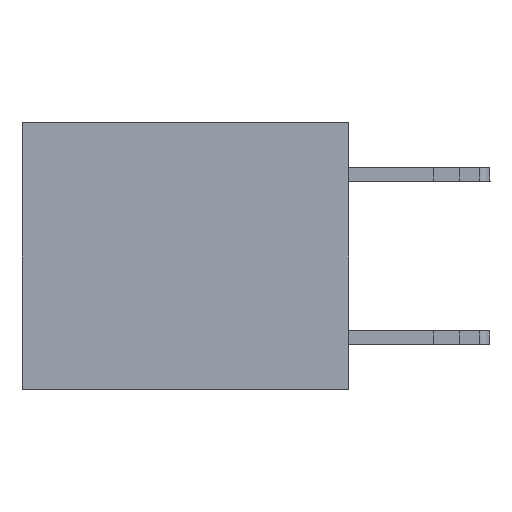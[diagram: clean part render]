
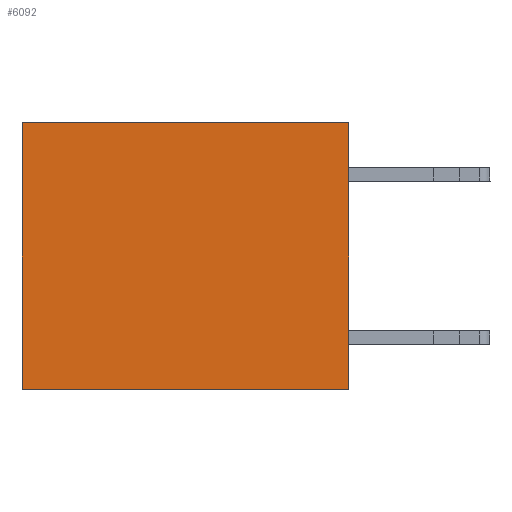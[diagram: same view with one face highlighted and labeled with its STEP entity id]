
A CAD part, left-side view. The second image highlights one B-rep face of the part: STEP entity #6092.
In plain terms, the highlighted planar face has unit normal (-1, 0, 0).
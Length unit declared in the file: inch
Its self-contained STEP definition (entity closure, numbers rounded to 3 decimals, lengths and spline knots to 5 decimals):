
#1588 = VERTEX_POINT ( 'NONE', #6888 ) ;
#2397 = EDGE_CURVE ( 'NONE', #4561, #4351, #5416, .T. ) ;
#2627 = CARTESIAN_POINT ( 'NONE',  ( 0.3165, 0., -0.49 ) ) ;
#3205 = VECTOR ( 'NONE', #15826, 39.37008 ) ;
#3655 = DIRECTION ( 'NONE',  ( 0., 0., -1. ) ) ;
#4344 = ORIENTED_EDGE ( 'NONE', *, *, #4669, .F. ) ;
#4351 = VERTEX_POINT ( 'NONE', #10273 ) ;
#4561 = VERTEX_POINT ( 'NONE', #13708 ) ;
#4669 = EDGE_CURVE ( 'NONE', #1588, #4351, #12256, .T. ) ;
#5416 = LINE ( 'NONE', #12578, #13364 ) ;
#5904 = EDGE_CURVE ( 'NONE', #9114, #1588, #15426, .T. ) ;
#6092 = ADVANCED_FACE ( 'NONE', ( #16741 ), #17981, .F. ) ;
#6888 = CARTESIAN_POINT ( 'NONE',  ( 0.3165, 0., -0.49 ) ) ;
#7157 = CARTESIAN_POINT ( 'NONE',  ( 0.3165, 0., -0.49 ) ) ;
#7184 = ORIENTED_EDGE ( 'NONE', *, *, #2397, .T. ) ;
#7293 = DIRECTION ( 'NONE',  ( 0., 1., 0. ) ) ;
#7505 = CARTESIAN_POINT ( 'NONE',  ( 0.3165, 0., 0. ) ) ;
#7849 = ORIENTED_EDGE ( 'NONE', *, *, #12343, .T. ) ;
#9114 = VERTEX_POINT ( 'NONE', #7505 ) ;
#10273 = CARTESIAN_POINT ( 'NONE',  ( 0.3165, 0.6, -0.49 ) ) ;
#10950 = DIRECTION ( 'NONE',  ( 0., 0., -1. ) ) ;
#11194 = LINE ( 'NONE', #15739, #19763 ) ;
#12256 = LINE ( 'NONE', #14098, #3205 ) ;
#12343 = EDGE_CURVE ( 'NONE', #9114, #4561, #11194, .T. ) ;
#12578 = CARTESIAN_POINT ( 'NONE',  ( 0.3165, 0.6, -0.49 ) ) ;
#13364 = VECTOR ( 'NONE', #10950, 39.37008 ) ;
#13708 = CARTESIAN_POINT ( 'NONE',  ( 0.3165, 0.6, 0. ) ) ;
#14098 = CARTESIAN_POINT ( 'NONE',  ( 0.3165, 0., -0.49 ) ) ;
#15426 = LINE ( 'NONE', #7157, #16499 ) ;
#15739 = CARTESIAN_POINT ( 'NONE',  ( 0.3165, 0., 0. ) ) ;
#15826 = DIRECTION ( 'NONE',  ( 0., 1., 0. ) ) ;
#16125 = DIRECTION ( 'NONE',  ( 0., 0., -1. ) ) ;
#16194 = EDGE_LOOP ( 'NONE', ( #7184, #4344, #18885, #7849 ) ) ;
#16499 = VECTOR ( 'NONE', #3655, 39.37008 ) ;
#16741 = FACE_OUTER_BOUND ( 'NONE', #16194, .T. ) ;
#16959 = AXIS2_PLACEMENT_3D ( 'NONE', #2627, #21402, #16125 ) ;
#17981 = PLANE ( 'NONE',  #16959 ) ;
#18885 = ORIENTED_EDGE ( 'NONE', *, *, #5904, .F. ) ;
#19763 = VECTOR ( 'NONE', #7293, 39.37008 ) ;
#21402 = DIRECTION ( 'NONE',  ( 1., 0., 0. ) ) ;
